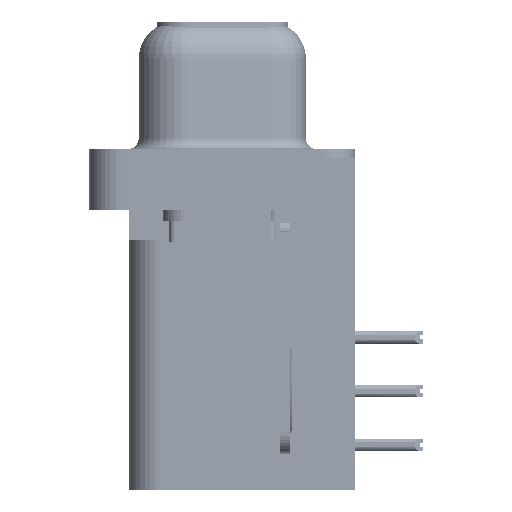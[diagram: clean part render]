
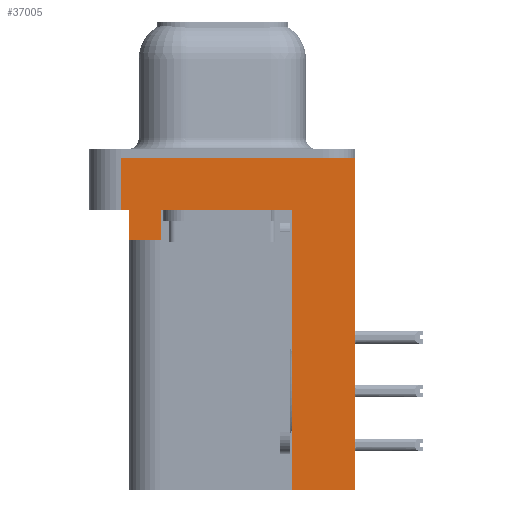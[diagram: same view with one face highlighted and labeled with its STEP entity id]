
A CAD part, left-side view. The second image highlights one B-rep face of the part: STEP entity #37005.
In plain terms, the highlighted planar face has unit normal (-1, 0, 0).
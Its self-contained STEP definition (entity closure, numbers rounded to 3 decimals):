
#1015 = VERTEX_POINT ( 'NONE', #7089 ) ;
#2005 = DIRECTION ( 'NONE',  ( 0., 0., 1. ) ) ;
#2272 = DIRECTION ( 'NONE',  ( 0., 0., 1. ) ) ;
#3587 = DIRECTION ( 'NONE',  ( 0., 1., 0. ) ) ;
#4198 = DIRECTION ( 'NONE',  ( 0., 0., 1. ) ) ;
#4779 = ORIENTED_EDGE ( 'NONE', *, *, #13331, .F. ) ;
#5129 = DIRECTION ( 'NONE',  ( 0., -1., 0. ) ) ;
#5513 = DIRECTION ( 'NONE',  ( -1., 0., 0. ) ) ;
#7089 = CARTESIAN_POINT ( 'NONE',  ( -2.91, -3.295, -15.7 ) ) ;
#9243 = CARTESIAN_POINT ( 'NONE',  ( -2.91, 2.895, -3.9 ) ) ;
#9344 = ORIENTED_EDGE ( 'NONE', *, *, #53488, .F. ) ;
#9921 = VERTEX_POINT ( 'NONE', #22493 ) ;
#10572 = VERTEX_POINT ( 'NONE', #32222 ) ;
#10681 = ORIENTED_EDGE ( 'NONE', *, *, #51433, .F. ) ;
#13147 = EDGE_CURVE ( 'NONE', #10572, #20670, #25830, .T. ) ;
#13331 = EDGE_CURVE ( 'NONE', #45035, #20670, #46101, .T. ) ;
#13524 = VECTOR ( 'NONE', #2272, 1000. ) ;
#13605 = CARTESIAN_POINT ( 'NONE',  ( -2.91, -6.275, -2.5 ) ) ;
#15680 = CARTESIAN_POINT ( 'NONE',  ( -2.91, 4.425, -2.5 ) ) ;
#17033 = VECTOR ( 'NONE', #3587, 1000. ) ;
#17353 = CARTESIAN_POINT ( 'NONE',  ( -2.91, 4.425, -3.9 ) ) ;
#19108 = DIRECTION ( 'NONE',  ( 0., -1., 0. ) ) ;
#19684 = ORIENTED_EDGE ( 'NONE', *, *, #44089, .T. ) ;
#20107 = VECTOR ( 'NONE', #5129, 1000. ) ;
#20512 = EDGE_CURVE ( 'NONE', #28974, #27812, #33502, .T. ) ;
#20670 = VERTEX_POINT ( 'NONE', #36827 ) ;
#21915 = VERTEX_POINT ( 'NONE', #17353 ) ;
#22493 = CARTESIAN_POINT ( 'NONE',  ( -2.91, 2.895, -3.9 ) ) ;
#23090 = CARTESIAN_POINT ( 'NONE',  ( -2.91, -6.275, -2.5 ) ) ;
#23434 = CARTESIAN_POINT ( 'NONE',  ( -2.91, -3.295, -15.7 ) ) ;
#24458 = CARTESIAN_POINT ( 'NONE',  ( -2.91, 4.425, -3.9 ) ) ;
#25253 = CARTESIAN_POINT ( 'NONE',  ( -2.91, 4.775, -2.5 ) ) ;
#25673 = CARTESIAN_POINT ( 'NONE',  ( -2.91, -6.275, 0. ) ) ;
#25830 = LINE ( 'NONE', #23090, #34375 ) ;
#25963 = FACE_OUTER_BOUND ( 'NONE', #35029, .T. ) ;
#26272 = VECTOR ( 'NONE', #26296, 1000. ) ;
#26296 = DIRECTION ( 'NONE',  ( 0., 0., 1. ) ) ;
#26984 = LINE ( 'NONE', #24458, #17033 ) ;
#27328 = VECTOR ( 'NONE', #27692, 1000. ) ;
#27601 = CARTESIAN_POINT ( 'NONE',  ( -2.91, 4.425, -3.9 ) ) ;
#27692 = DIRECTION ( 'NONE',  ( 0., 1., 0. ) ) ;
#27812 = VERTEX_POINT ( 'NONE', #39465 ) ;
#28109 = VECTOR ( 'NONE', #4198, 1000. ) ;
#28656 = ORIENTED_EDGE ( 'NONE', *, *, #20512, .T. ) ;
#28974 = VERTEX_POINT ( 'NONE', #46612 ) ;
#29035 = EDGE_CURVE ( 'NONE', #9921, #28974, #37460, .T. ) ;
#29897 = DIRECTION ( 'NONE',  ( 0., -1., 0. ) ) ;
#30046 = LINE ( 'NONE', #13605, #20107 ) ;
#30062 = CARTESIAN_POINT ( 'NONE',  ( -2.91, 4.775, -2.5 ) ) ;
#30785 = CARTESIAN_POINT ( 'NONE',  ( -2.91, -6.275, -2.5 ) ) ;
#31657 = ORIENTED_EDGE ( 'NONE', *, *, #53783, .F. ) ;
#32222 = CARTESIAN_POINT ( 'NONE',  ( -2.91, -6.275, -15.7 ) ) ;
#33502 = LINE ( 'NONE', #40122, #34839 ) ;
#33591 = DIRECTION ( 'NONE',  ( 0., 0., 1. ) ) ;
#34375 = VECTOR ( 'NONE', #2005, 1000. ) ;
#34839 = VECTOR ( 'NONE', #19108, 1000. ) ;
#35011 = VECTOR ( 'NONE', #29897, 1000. ) ;
#35019 = DIRECTION ( 'NONE',  ( 0., 0., 1. ) ) ;
#35029 = EDGE_LOOP ( 'NONE', ( #4779, #10681, #19684, #53883, #39926, #53977, #28656, #9344, #31657, #37341 ) ) ;
#36562 = VECTOR ( 'NONE', #33591, 1000. ) ;
#36587 = VERTEX_POINT ( 'NONE', #15680 ) ;
#36827 = CARTESIAN_POINT ( 'NONE',  ( -2.91, -6.275, 0. ) ) ;
#36844 = VERTEX_POINT ( 'NONE', #30062 ) ;
#37005 = ADVANCED_FACE ( 'NONE', ( #25963 ), #47428, .T. ) ;
#37341 = ORIENTED_EDGE ( 'NONE', *, *, #13147, .T. ) ;
#37460 = LINE ( 'NONE', #9243, #26272 ) ;
#37971 = LINE ( 'NONE', #25253, #28109 ) ;
#38497 = LINE ( 'NONE', #23434, #27328 ) ;
#39465 = CARTESIAN_POINT ( 'NONE',  ( -2.91, -3.295, -2.5 ) ) ;
#39926 = ORIENTED_EDGE ( 'NONE', *, *, #40621, .F. ) ;
#40122 = CARTESIAN_POINT ( 'NONE',  ( -2.91, -6.275, -2.5 ) ) ;
#40621 = EDGE_CURVE ( 'NONE', #9921, #21915, #26984, .T. ) ;
#44089 = EDGE_CURVE ( 'NONE', #36844, #36587, #30046, .T. ) ;
#45035 = VERTEX_POINT ( 'NONE', #49332 ) ;
#45384 = AXIS2_PLACEMENT_3D ( 'NONE', #30785, #5513, #35019 ) ;
#46101 = LINE ( 'NONE', #25673, #35011 ) ;
#46612 = CARTESIAN_POINT ( 'NONE',  ( -2.91, 2.895, -2.5 ) ) ;
#47428 = PLANE ( 'NONE',  #45384 ) ;
#47638 = LINE ( 'NONE', #50394, #36562 ) ;
#48361 = LINE ( 'NONE', #27601, #13524 ) ;
#49332 = CARTESIAN_POINT ( 'NONE',  ( -2.91, 4.775, 0. ) ) ;
#50394 = CARTESIAN_POINT ( 'NONE',  ( -2.91, -3.295, -15.7 ) ) ;
#51433 = EDGE_CURVE ( 'NONE', #36844, #45035, #37971, .T. ) ;
#51753 = EDGE_CURVE ( 'NONE', #21915, #36587, #48361, .T. ) ;
#53488 = EDGE_CURVE ( 'NONE', #1015, #27812, #47638, .T. ) ;
#53783 = EDGE_CURVE ( 'NONE', #10572, #1015, #38497, .T. ) ;
#53883 = ORIENTED_EDGE ( 'NONE', *, *, #51753, .F. ) ;
#53977 = ORIENTED_EDGE ( 'NONE', *, *, #29035, .T. ) ;
